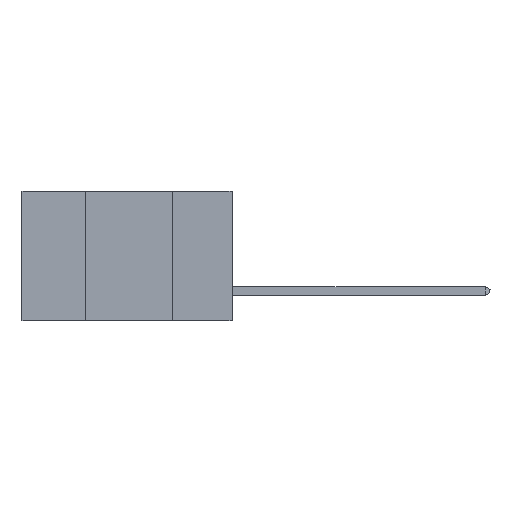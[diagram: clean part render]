
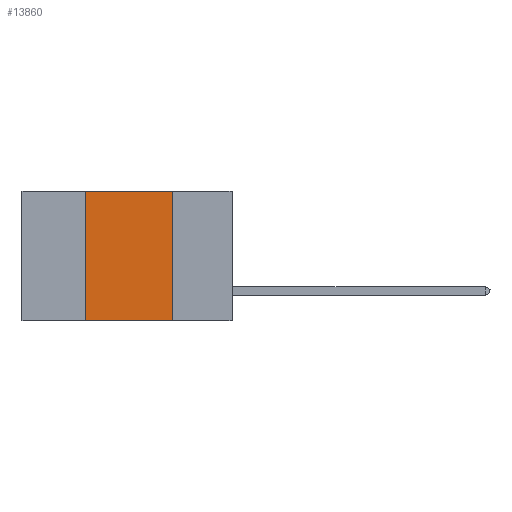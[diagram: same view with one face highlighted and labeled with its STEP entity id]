
A CAD part, left-side view. The second image highlights one B-rep face of the part: STEP entity #13860.
In plain terms, the highlighted planar face has unit normal (-1, 0, 0).
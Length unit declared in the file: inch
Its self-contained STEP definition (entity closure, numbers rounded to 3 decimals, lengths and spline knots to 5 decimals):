
#44 = CARTESIAN_POINT ( 'NONE',  ( 0., 0.42, 0. ) ) ;
#233 = DIRECTION ( 'NONE',  ( 1., 0., 0. ) ) ;
#844 = FACE_OUTER_BOUND ( 'NONE', #13815, .T. ) ;
#1549 = ORIENTED_EDGE ( 'NONE', *, *, #15395, .F. ) ;
#1698 = CARTESIAN_POINT ( 'NONE',  ( 0., 0.6, 0. ) ) ;
#1717 = DIRECTION ( 'NONE',  ( 0., 0., -1. ) ) ;
#1984 = VERTEX_POINT ( 'NONE', #7297 ) ;
#2444 = VECTOR ( 'NONE', #18039, 39.37008 ) ;
#3106 = CARTESIAN_POINT ( 'NONE',  ( 0., 0.6, -0.37 ) ) ;
#3375 = LINE ( 'NONE', #3106, #2444 ) ;
#4483 = EDGE_CURVE ( 'NONE', #7108, #13530, #3375, .T. ) ;
#4575 = ORIENTED_EDGE ( 'NONE', *, *, #10509, .F. ) ;
#7108 = VERTEX_POINT ( 'NONE', #17223 ) ;
#7231 = LINE ( 'NONE', #44, #18377 ) ;
#7297 = CARTESIAN_POINT ( 'NONE',  ( 0., 0.42, 0. ) ) ;
#8649 = AXIS2_PLACEMENT_3D ( 'NONE', #9114, #233, #1717 ) ;
#9114 = CARTESIAN_POINT ( 'NONE',  ( 0., 0.6, 0. ) ) ;
#9675 = CARTESIAN_POINT ( 'NONE',  ( 0., 0.17, 0. ) ) ;
#9740 = ORIENTED_EDGE ( 'NONE', *, *, #14301, .F. ) ;
#10509 = EDGE_CURVE ( 'NONE', #7108, #1984, #7231, .T. ) ;
#10672 = CARTESIAN_POINT ( 'NONE',  ( 0., 0.17, -0.37 ) ) ;
#11522 = VERTEX_POINT ( 'NONE', #9675 ) ;
#13302 = DIRECTION ( 'NONE',  ( 0., -1., 0. ) ) ;
#13530 = VERTEX_POINT ( 'NONE', #10672 ) ;
#13815 = EDGE_LOOP ( 'NONE', ( #9740, #1549, #4575, #18677 ) ) ;
#13860 = ADVANCED_FACE ( 'NONE', ( #844 ), #13917, .F. ) ;
#13917 = PLANE ( 'NONE',  #8649 ) ;
#14301 = EDGE_CURVE ( 'NONE', #11522, #13530, #15292, .T. ) ;
#15118 = DIRECTION ( 'NONE',  ( 0., 0., -1. ) ) ;
#15292 = LINE ( 'NONE', #17841, #15530 ) ;
#15395 = EDGE_CURVE ( 'NONE', #1984, #11522, #18103, .T. ) ;
#15530 = VECTOR ( 'NONE', #15118, 39.37008 ) ;
#16411 = DIRECTION ( 'NONE',  ( 0., 0., 1. ) ) ;
#16733 = VECTOR ( 'NONE', #13302, 39.37008 ) ;
#17223 = CARTESIAN_POINT ( 'NONE',  ( 0., 0.42, -0.37 ) ) ;
#17841 = CARTESIAN_POINT ( 'NONE',  ( 0., 0.17, 0. ) ) ;
#18039 = DIRECTION ( 'NONE',  ( 0., -1., 0. ) ) ;
#18103 = LINE ( 'NONE', #1698, #16733 ) ;
#18377 = VECTOR ( 'NONE', #16411, 39.37008 ) ;
#18677 = ORIENTED_EDGE ( 'NONE', *, *, #4483, .T. ) ;
